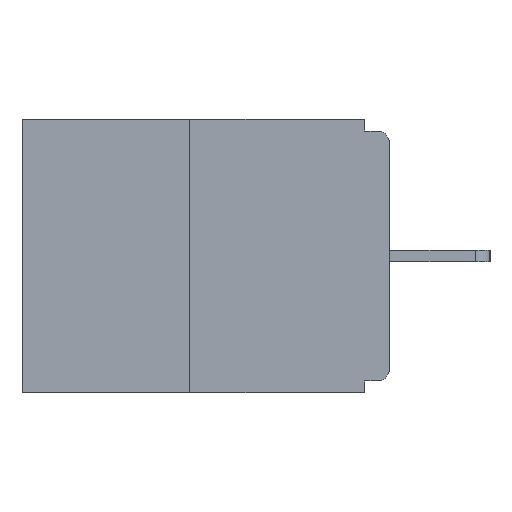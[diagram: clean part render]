
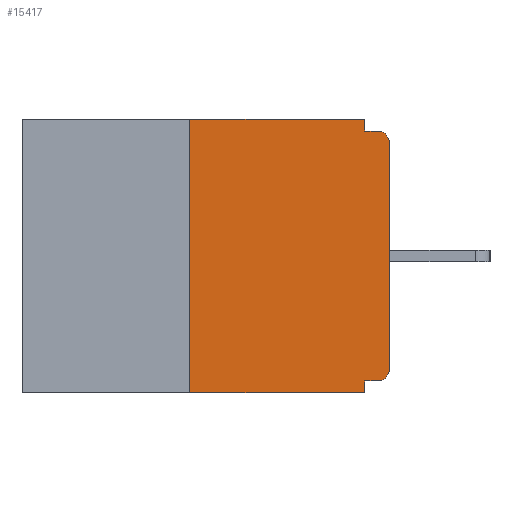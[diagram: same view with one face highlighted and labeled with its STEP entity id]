
A CAD part, left-side view. The second image highlights one B-rep face of the part: STEP entity #15417.
In plain terms, the highlighted planar face has unit normal (-1, 0, 0).
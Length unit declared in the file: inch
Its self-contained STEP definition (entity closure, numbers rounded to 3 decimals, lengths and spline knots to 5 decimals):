
#119 = VECTOR ( 'NONE', #17485, 39.37008 ) ;
#782 = VECTOR ( 'NONE', #11869, 39.37008 ) ;
#1079 = CARTESIAN_POINT ( 'NONE',  ( 0., 0.46, 0. ) ) ;
#1295 = EDGE_CURVE ( 'NONE', #8856, #18865, #2974, .T. ) ;
#1382 = CARTESIAN_POINT ( 'NONE',  ( 0., 0.031, 0. ) ) ;
#1522 = DIRECTION ( 'NONE',  ( 0., 1., 0. ) ) ;
#1796 = VERTEX_POINT ( 'NONE', #15283 ) ;
#1797 = CARTESIAN_POINT ( 'NONE',  ( 0., 0.031, 0. ) ) ;
#1919 = VERTEX_POINT ( 'NONE', #14496 ) ;
#2150 = VECTOR ( 'NONE', #11958, 39.37008 ) ;
#2200 = DIRECTION ( 'NONE',  ( -1., 0., 0. ) ) ;
#2573 = VECTOR ( 'NONE', #12936, 39.37008 ) ;
#2576 = CARTESIAN_POINT ( 'NONE',  ( 0., 0., 0. ) ) ;
#2791 = EDGE_CURVE ( 'NONE', #12146, #1919, #17373, .T. ) ;
#2974 = LINE ( 'NONE', #5939, #2150 ) ;
#3104 = VECTOR ( 'NONE', #11747, 39.37008 ) ;
#3229 = LINE ( 'NONE', #9238, #4547 ) ;
#3389 = CARTESIAN_POINT ( 'NONE',  ( 0., 0.25, -0.343 ) ) ;
#4372 = EDGE_CURVE ( 'NONE', #1796, #12146, #5389, .T. ) ;
#4419 = CARTESIAN_POINT ( 'NONE',  ( 0., 0.015, -0.015 ) ) ;
#4480 = CARTESIAN_POINT ( 'NONE',  ( 0., 0.25, 0. ) ) ;
#4547 = VECTOR ( 'NONE', #7766, 39.37008 ) ;
#4684 = DIRECTION ( 'NONE',  ( 0., 0., -1. ) ) ;
#4820 = ORIENTED_EDGE ( 'NONE', *, *, #9727, .F. ) ;
#4909 = VERTEX_POINT ( 'NONE', #1797 ) ;
#5087 = VECTOR ( 'NONE', #1522, 39.37008 ) ;
#5389 = CIRCLE ( 'NONE', #8217, 0.015 ) ;
#5744 = CARTESIAN_POINT ( 'NONE',  ( 0., 0., -0.313 ) ) ;
#5917 = LINE ( 'NONE', #1382, #3104 ) ;
#5939 = CARTESIAN_POINT ( 'NONE',  ( 0., 0., -0.015 ) ) ;
#5942 = EDGE_CURVE ( 'NONE', #1796, #14649, #14941, .T. ) ;
#6045 = CARTESIAN_POINT ( 'NONE',  ( 0., 0.031, -0.343 ) ) ;
#6243 = EDGE_CURVE ( 'NONE', #1919, #18865, #18017, .T. ) ;
#6817 = ORIENTED_EDGE ( 'NONE', *, *, #6243, .T. ) ;
#6909 = ORIENTED_EDGE ( 'NONE', *, *, #13721, .F. ) ;
#7084 = FACE_OUTER_BOUND ( 'NONE', #9580, .T. ) ;
#7088 = ORIENTED_EDGE ( 'NONE', *, *, #1295, .F. ) ;
#7463 = DIRECTION ( 'NONE',  ( 1., 0., 0. ) ) ;
#7502 = EDGE_CURVE ( 'NONE', #18381, #11928, #17588, .T. ) ;
#7766 = DIRECTION ( 'NONE',  ( 0., 0., 1. ) ) ;
#7902 = DIRECTION ( 'NONE',  ( 0., -1., 0. ) ) ;
#8217 = AXIS2_PLACEMENT_3D ( 'NONE', #19281, #10893, #4684 ) ;
#8649 = EDGE_CURVE ( 'NONE', #14649, #11928, #17890, .T. ) ;
#8717 = CARTESIAN_POINT ( 'NONE',  ( 0., 0., -0.328 ) ) ;
#8856 = VERTEX_POINT ( 'NONE', #9396 ) ;
#9238 = CARTESIAN_POINT ( 'NONE',  ( 0., 0.25, 0. ) ) ;
#9396 = CARTESIAN_POINT ( 'NONE',  ( 0., 0.031, -0.015 ) ) ;
#9580 = EDGE_LOOP ( 'NONE', ( #10684, #4820, #15800, #10532, #17471, #9591, #11481, #6817, #7088, #6909 ) ) ;
#9591 = ORIENTED_EDGE ( 'NONE', *, *, #4372, .T. ) ;
#9665 = LINE ( 'NONE', #18441, #13708 ) ;
#9727 = EDGE_CURVE ( 'NONE', #18381, #11559, #3229, .T. ) ;
#10142 = DIRECTION ( 'NONE',  ( 0., 0., -1. ) ) ;
#10432 = EDGE_CURVE ( 'NONE', #11559, #4909, #9665, .T. ) ;
#10532 = ORIENTED_EDGE ( 'NONE', *, *, #8649, .F. ) ;
#10684 = ORIENTED_EDGE ( 'NONE', *, *, #10432, .F. ) ;
#10893 = DIRECTION ( 'NONE',  ( -1., 0., 0. ) ) ;
#11481 = ORIENTED_EDGE ( 'NONE', *, *, #2791, .T. ) ;
#11559 = VERTEX_POINT ( 'NONE', #4480 ) ;
#11747 = DIRECTION ( 'NONE',  ( 0., 0., -1. ) ) ;
#11869 = DIRECTION ( 'NONE',  ( 0., 0., -1. ) ) ;
#11928 = VERTEX_POINT ( 'NONE', #14052 ) ;
#11958 = DIRECTION ( 'NONE',  ( 0., -1., 0. ) ) ;
#12146 = VERTEX_POINT ( 'NONE', #5744 ) ;
#12745 = CARTESIAN_POINT ( 'NONE',  ( 0., 0.015, -0.03 ) ) ;
#12936 = DIRECTION ( 'NONE',  ( 0., 0., 1. ) ) ;
#13314 = AXIS2_PLACEMENT_3D ( 'NONE', #12745, #2200, #14338 ) ;
#13391 = PLANE ( 'NONE',  #15076 ) ;
#13446 = CARTESIAN_POINT ( 'NONE',  ( 0., 0.031, -0.328 ) ) ;
#13708 = VECTOR ( 'NONE', #7902, 39.37008 ) ;
#13721 = EDGE_CURVE ( 'NONE', #4909, #8856, #5917, .T. ) ;
#14052 = CARTESIAN_POINT ( 'NONE',  ( 0., 0.031, -0.343 ) ) ;
#14338 = DIRECTION ( 'NONE',  ( 0., 0., -1. ) ) ;
#14496 = CARTESIAN_POINT ( 'NONE',  ( 0., 0., -0.03 ) ) ;
#14649 = VERTEX_POINT ( 'NONE', #13446 ) ;
#14941 = LINE ( 'NONE', #8717, #5087 ) ;
#15076 = AXIS2_PLACEMENT_3D ( 'NONE', #1079, #7463, #10142 ) ;
#15283 = CARTESIAN_POINT ( 'NONE',  ( 0., 0.015, -0.328 ) ) ;
#15417 = ADVANCED_FACE ( 'NONE', ( #7084 ), #13391, .F. ) ;
#15713 = CARTESIAN_POINT ( 'NONE',  ( 0., 0.46, -0.343 ) ) ;
#15800 = ORIENTED_EDGE ( 'NONE', *, *, #7502, .T. ) ;
#17373 = LINE ( 'NONE', #2576, #2573 ) ;
#17471 = ORIENTED_EDGE ( 'NONE', *, *, #5942, .F. ) ;
#17485 = DIRECTION ( 'NONE',  ( 0., -1., 0. ) ) ;
#17588 = LINE ( 'NONE', #15713, #119 ) ;
#17890 = LINE ( 'NONE', #6045, #782 ) ;
#18017 = CIRCLE ( 'NONE', #13314, 0.015 ) ;
#18381 = VERTEX_POINT ( 'NONE', #3389 ) ;
#18441 = CARTESIAN_POINT ( 'NONE',  ( 0., 0.46, 0. ) ) ;
#18865 = VERTEX_POINT ( 'NONE', #4419 ) ;
#19281 = CARTESIAN_POINT ( 'NONE',  ( 0., 0.015, -0.313 ) ) ;
